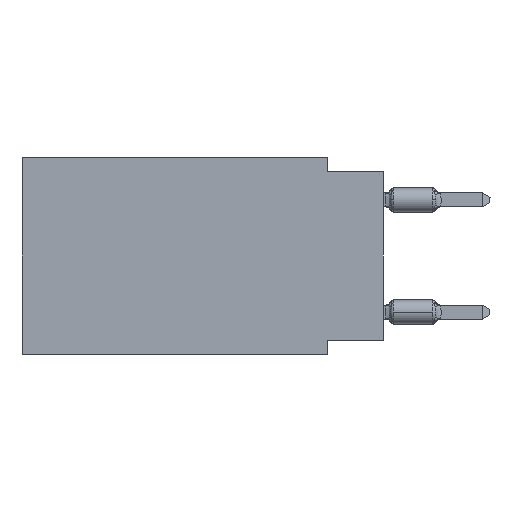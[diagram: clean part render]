
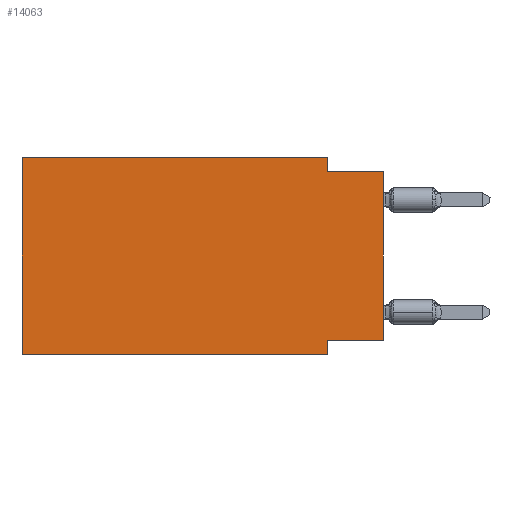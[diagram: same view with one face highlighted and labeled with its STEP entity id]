
A CAD part, left-side view. The second image highlights one B-rep face of the part: STEP entity #14063.
In plain terms, the highlighted planar face has unit normal (-1, 0, 0).
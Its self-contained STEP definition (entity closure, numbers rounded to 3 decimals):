
#1152 = CARTESIAN_POINT ( 'NONE',  ( 0., 2.54, 0. ) ) ;
#1257 = CARTESIAN_POINT ( 'NONE',  ( 0., 16.383, -8.89 ) ) ;
#1859 = PLANE ( 'NONE',  #6935 ) ;
#2091 = CARTESIAN_POINT ( 'NONE',  ( 0., 0., -8.255 ) ) ;
#2118 = CARTESIAN_POINT ( 'NONE',  ( 0., 0., 0. ) ) ;
#2276 = DIRECTION ( 'NONE',  ( 0., 0., 1. ) ) ;
#2650 = ORIENTED_EDGE ( 'NONE', *, *, #17803, .F. ) ;
#2779 = VERTEX_POINT ( 'NONE', #27883 ) ;
#3422 = LINE ( 'NONE', #13295, #18568 ) ;
#3494 = DIRECTION ( 'NONE',  ( 0., -1., 0. ) ) ;
#3503 = CARTESIAN_POINT ( 'NONE',  ( 0., 16.383, -8.89 ) ) ;
#3680 = LINE ( 'NONE', #1257, #18780 ) ;
#3905 = VERTEX_POINT ( 'NONE', #7450 ) ;
#3972 = DIRECTION ( 'NONE',  ( 1., 0., 0. ) ) ;
#4263 = CARTESIAN_POINT ( 'NONE',  ( 0., 16.383, 0. ) ) ;
#5545 = DIRECTION ( 'NONE',  ( 0., 0., 1. ) ) ;
#6153 = DIRECTION ( 'NONE',  ( 0., 0., -1. ) ) ;
#6935 = AXIS2_PLACEMENT_3D ( 'NONE', #11252, #3972, #21161 ) ;
#7121 = EDGE_CURVE ( 'NONE', #12294, #14901, #16879, .T. ) ;
#7450 = CARTESIAN_POINT ( 'NONE',  ( 0., 2.54, 0. ) ) ;
#8340 = LINE ( 'NONE', #25722, #20045 ) ;
#8524 = DIRECTION ( 'NONE',  ( 0., -1., 0. ) ) ;
#9382 = DIRECTION ( 'NONE',  ( 0., 1., 0. ) ) ;
#9435 = VECTOR ( 'NONE', #9382, 1000. ) ;
#10047 = ORIENTED_EDGE ( 'NONE', *, *, #25460, .F. ) ;
#10103 = CARTESIAN_POINT ( 'NONE',  ( 0., 2.54, -8.89 ) ) ;
#10267 = EDGE_CURVE ( 'NONE', #27254, #21004, #25040, .T. ) ;
#10461 = EDGE_LOOP ( 'NONE', ( #17764, #10682, #10047, #2650, #18660, #12365, #22072, #18878 ) ) ;
#10682 = ORIENTED_EDGE ( 'NONE', *, *, #16839, .F. ) ;
#11252 = CARTESIAN_POINT ( 'NONE',  ( 0., 16.383, 0. ) ) ;
#12294 = VERTEX_POINT ( 'NONE', #21883 ) ;
#12365 = ORIENTED_EDGE ( 'NONE', *, *, #25669, .T. ) ;
#12839 = CARTESIAN_POINT ( 'NONE',  ( 0., 16.383, 0. ) ) ;
#13295 = CARTESIAN_POINT ( 'NONE',  ( 0., 2.54, -8.89 ) ) ;
#13547 = CARTESIAN_POINT ( 'NONE',  ( 0., 0., -0.635 ) ) ;
#14063 = ADVANCED_FACE ( 'NONE', ( #23928 ), #1859, .F. ) ;
#14901 = VERTEX_POINT ( 'NONE', #29819 ) ;
#15949 = EDGE_CURVE ( 'NONE', #2779, #17110, #3422, .T. ) ;
#16307 = VERTEX_POINT ( 'NONE', #22667 ) ;
#16839 = EDGE_CURVE ( 'NONE', #16307, #14901, #31397, .T. ) ;
#16879 = LINE ( 'NONE', #2118, #29576 ) ;
#17110 = VERTEX_POINT ( 'NONE', #10103 ) ;
#17764 = ORIENTED_EDGE ( 'NONE', *, *, #7121, .T. ) ;
#17803 = EDGE_CURVE ( 'NONE', #21004, #3905, #8340, .T. ) ;
#18101 = VECTOR ( 'NONE', #8524, 1000. ) ;
#18568 = VECTOR ( 'NONE', #27750, 1000. ) ;
#18660 = ORIENTED_EDGE ( 'NONE', *, *, #10267, .F. ) ;
#18780 = VECTOR ( 'NONE', #28658, 1000. ) ;
#18878 = ORIENTED_EDGE ( 'NONE', *, *, #26617, .F. ) ;
#19308 = VECTOR ( 'NONE', #6153, 1000. ) ;
#20045 = VECTOR ( 'NONE', #3494, 1000. ) ;
#20932 = LINE ( 'NONE', #1152, #19308 ) ;
#21004 = VERTEX_POINT ( 'NONE', #4263 ) ;
#21161 = DIRECTION ( 'NONE',  ( 0., 0., -1. ) ) ;
#21565 = LINE ( 'NONE', #2091, #9435 ) ;
#21883 = CARTESIAN_POINT ( 'NONE',  ( 0., 0., -8.255 ) ) ;
#22072 = ORIENTED_EDGE ( 'NONE', *, *, #15949, .F. ) ;
#22667 = CARTESIAN_POINT ( 'NONE',  ( 0., 2.54, -0.635 ) ) ;
#23928 = FACE_OUTER_BOUND ( 'NONE', #10461, .T. ) ;
#25040 = LINE ( 'NONE', #12839, #29010 ) ;
#25460 = EDGE_CURVE ( 'NONE', #3905, #16307, #20932, .T. ) ;
#25669 = EDGE_CURVE ( 'NONE', #27254, #17110, #3680, .T. ) ;
#25722 = CARTESIAN_POINT ( 'NONE',  ( 0., 16.383, 0. ) ) ;
#26617 = EDGE_CURVE ( 'NONE', #12294, #2779, #21565, .T. ) ;
#27254 = VERTEX_POINT ( 'NONE', #3503 ) ;
#27750 = DIRECTION ( 'NONE',  ( 0., 0., -1. ) ) ;
#27883 = CARTESIAN_POINT ( 'NONE',  ( 0., 2.54, -8.255 ) ) ;
#28658 = DIRECTION ( 'NONE',  ( 0., -1., 0. ) ) ;
#29010 = VECTOR ( 'NONE', #5545, 1000. ) ;
#29576 = VECTOR ( 'NONE', #2276, 1000. ) ;
#29819 = CARTESIAN_POINT ( 'NONE',  ( 0., 0., -0.635 ) ) ;
#31397 = LINE ( 'NONE', #13547, #18101 ) ;
